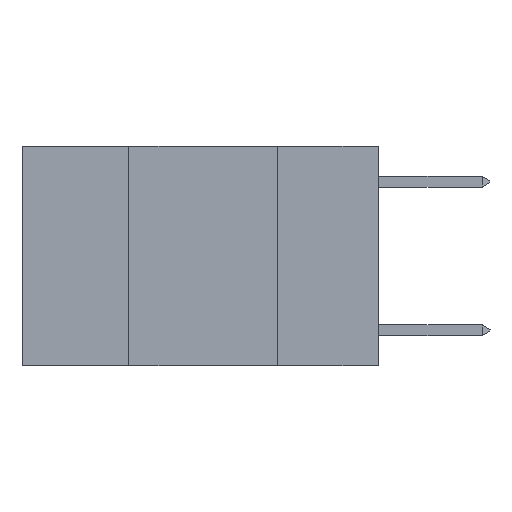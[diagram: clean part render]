
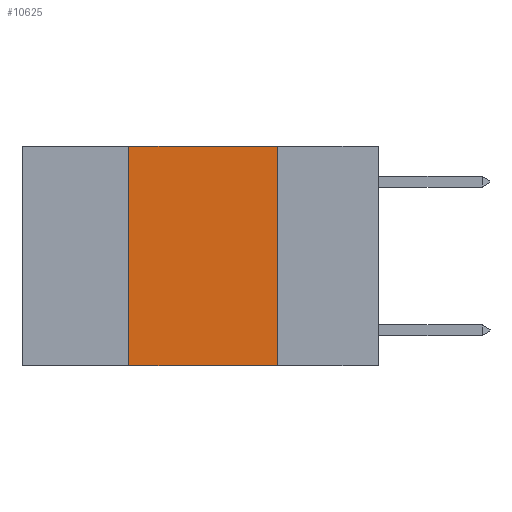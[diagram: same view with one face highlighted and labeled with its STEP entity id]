
A CAD part, left-side view. The second image highlights one B-rep face of the part: STEP entity #10625.
In plain terms, the highlighted planar face has unit normal (-1, 0, 0).
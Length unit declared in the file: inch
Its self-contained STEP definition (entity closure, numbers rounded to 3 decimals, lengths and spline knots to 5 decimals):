
#681 = CARTESIAN_POINT ( 'NONE',  ( 0., 0.42, -0.37 ) ) ;
#1722 = VECTOR ( 'NONE', #17130, 39.37008 ) ;
#2632 = VECTOR ( 'NONE', #13072, 39.37008 ) ;
#3086 = CARTESIAN_POINT ( 'NONE',  ( 0., 0.6, 0. ) ) ;
#3241 = CARTESIAN_POINT ( 'NONE',  ( 0., 0.42, 0. ) ) ;
#3345 = DIRECTION ( 'NONE',  ( 0., 0., -1. ) ) ;
#3381 = DIRECTION ( 'NONE',  ( 1., 0., 0. ) ) ;
#3528 = PLANE ( 'NONE',  #12264 ) ;
#3645 = CARTESIAN_POINT ( 'NONE',  ( 0., 0.6, 0. ) ) ;
#4005 = EDGE_CURVE ( 'NONE', #14316, #12777, #16767, .T. ) ;
#4300 = CARTESIAN_POINT ( 'NONE',  ( 0., 0.17, 0. ) ) ;
#4859 = VERTEX_POINT ( 'NONE', #8720 ) ;
#8720 = CARTESIAN_POINT ( 'NONE',  ( 0., 0.17, -0.37 ) ) ;
#9263 = FACE_OUTER_BOUND ( 'NONE', #18021, .T. ) ;
#10091 = VECTOR ( 'NONE', #18117, 39.37008 ) ;
#10544 = LINE ( 'NONE', #16707, #10091 ) ;
#10557 = VERTEX_POINT ( 'NONE', #4300 ) ;
#10625 = ADVANCED_FACE ( 'NONE', ( #9263 ), #3528, .F. ) ;
#11742 = CARTESIAN_POINT ( 'NONE',  ( 0., 0.6, -0.37 ) ) ;
#11814 = ORIENTED_EDGE ( 'NONE', *, *, #11901, .F. ) ;
#11901 = EDGE_CURVE ( 'NONE', #10557, #4859, #10544, .T. ) ;
#11976 = ORIENTED_EDGE ( 'NONE', *, *, #12108, .F. ) ;
#12012 = ORIENTED_EDGE ( 'NONE', *, *, #4005, .F. ) ;
#12108 = EDGE_CURVE ( 'NONE', #12777, #10557, #14012, .T. ) ;
#12173 = ORIENTED_EDGE ( 'NONE', *, *, #15426, .T. ) ;
#12264 = AXIS2_PLACEMENT_3D ( 'NONE', #3645, #3381, #3345 ) ;
#12777 = VERTEX_POINT ( 'NONE', #3241 ) ;
#13072 = DIRECTION ( 'NONE',  ( 0., -1., 0. ) ) ;
#13133 = DIRECTION ( 'NONE',  ( 0., -1., 0. ) ) ;
#13385 = VECTOR ( 'NONE', #13133, 39.37008 ) ;
#14012 = LINE ( 'NONE', #3086, #2632 ) ;
#14316 = VERTEX_POINT ( 'NONE', #681 ) ;
#15426 = EDGE_CURVE ( 'NONE', #14316, #4859, #18318, .T. ) ;
#16707 = CARTESIAN_POINT ( 'NONE',  ( 0., 0.17, 0. ) ) ;
#16767 = LINE ( 'NONE', #17083, #1722 ) ;
#17083 = CARTESIAN_POINT ( 'NONE',  ( 0., 0.42, 0. ) ) ;
#17130 = DIRECTION ( 'NONE',  ( 0., 0., 1. ) ) ;
#18021 = EDGE_LOOP ( 'NONE', ( #11814, #11976, #12012, #12173 ) ) ;
#18117 = DIRECTION ( 'NONE',  ( 0., 0., -1. ) ) ;
#18318 = LINE ( 'NONE', #11742, #13385 ) ;
